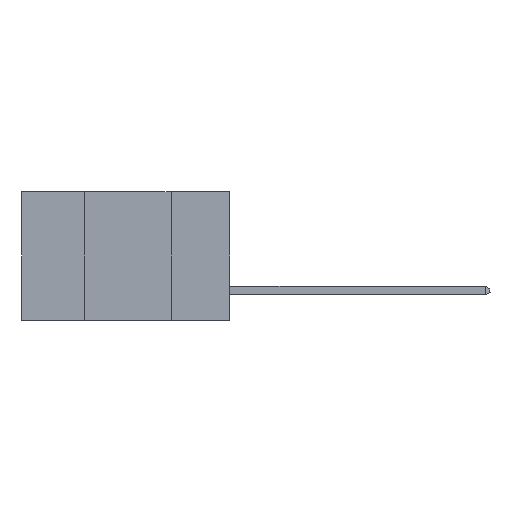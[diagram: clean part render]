
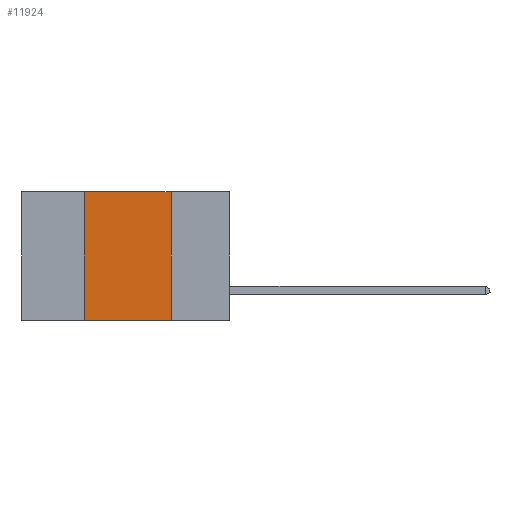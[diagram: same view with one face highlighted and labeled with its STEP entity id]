
A CAD part, left-side view. The second image highlights one B-rep face of the part: STEP entity #11924.
In plain terms, the highlighted planar face has unit normal (-1, 0, 0).
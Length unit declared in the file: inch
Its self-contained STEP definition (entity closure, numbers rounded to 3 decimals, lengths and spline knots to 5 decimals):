
#164 = EDGE_LOOP ( 'NONE', ( #11761, #11809, #6525, #10829 ) ) ;
#591 = AXIS2_PLACEMENT_3D ( 'NONE', #7668, #5528, #10982 ) ;
#1631 = CARTESIAN_POINT ( 'NONE',  ( 0., 0.17, -0.37 ) ) ;
#2065 = FACE_OUTER_BOUND ( 'NONE', #164, .T. ) ;
#2785 = CARTESIAN_POINT ( 'NONE',  ( 0., 0.17, 0. ) ) ;
#3423 = PLANE ( 'NONE',  #591 ) ;
#4293 = VECTOR ( 'NONE', #9358, 39.37008 ) ;
#4416 = VECTOR ( 'NONE', #4982, 39.37008 ) ;
#4982 = DIRECTION ( 'NONE',  ( 0., 0., -1. ) ) ;
#5528 = DIRECTION ( 'NONE',  ( 1., 0., 0. ) ) ;
#6487 = CARTESIAN_POINT ( 'NONE',  ( 0., 0.42, 0. ) ) ;
#6491 = LINE ( 'NONE', #7537, #8543 ) ;
#6525 = ORIENTED_EDGE ( 'NONE', *, *, #10486, .F. ) ;
#6785 = LINE ( 'NONE', #2785, #4416 ) ;
#7078 = CARTESIAN_POINT ( 'NONE',  ( 0., 0.42, 0. ) ) ;
#7537 = CARTESIAN_POINT ( 'NONE',  ( 0., 0.6, 0. ) ) ;
#7668 = CARTESIAN_POINT ( 'NONE',  ( 0., 0.6, 0. ) ) ;
#8543 = VECTOR ( 'NONE', #13131, 39.37008 ) ;
#8597 = VERTEX_POINT ( 'NONE', #6487 ) ;
#8600 = CARTESIAN_POINT ( 'NONE',  ( 0., 0.6, -0.37 ) ) ;
#9358 = DIRECTION ( 'NONE',  ( 0., 0., 1. ) ) ;
#9517 = VERTEX_POINT ( 'NONE', #9921 ) ;
#9609 = EDGE_CURVE ( 'NONE', #8597, #9517, #6491, .T. ) ;
#9921 = CARTESIAN_POINT ( 'NONE',  ( 0., 0.17, 0. ) ) ;
#10136 = EDGE_CURVE ( 'NONE', #11589, #12576, #10550, .T. ) ;
#10486 = EDGE_CURVE ( 'NONE', #11589, #8597, #10532, .T. ) ;
#10532 = LINE ( 'NONE', #7078, #4293 ) ;
#10550 = LINE ( 'NONE', #8600, #12947 ) ;
#10705 = CARTESIAN_POINT ( 'NONE',  ( 0., 0.42, -0.37 ) ) ;
#10829 = ORIENTED_EDGE ( 'NONE', *, *, #10136, .T. ) ;
#10982 = DIRECTION ( 'NONE',  ( 0., 0., -1. ) ) ;
#11566 = EDGE_CURVE ( 'NONE', #9517, #12576, #6785, .T. ) ;
#11589 = VERTEX_POINT ( 'NONE', #10705 ) ;
#11761 = ORIENTED_EDGE ( 'NONE', *, *, #11566, .F. ) ;
#11809 = ORIENTED_EDGE ( 'NONE', *, *, #9609, .F. ) ;
#11924 = ADVANCED_FACE ( 'NONE', ( #2065 ), #3423, .F. ) ;
#12067 = DIRECTION ( 'NONE',  ( 0., -1., 0. ) ) ;
#12576 = VERTEX_POINT ( 'NONE', #1631 ) ;
#12947 = VECTOR ( 'NONE', #12067, 39.37008 ) ;
#13131 = DIRECTION ( 'NONE',  ( 0., -1., 0. ) ) ;
